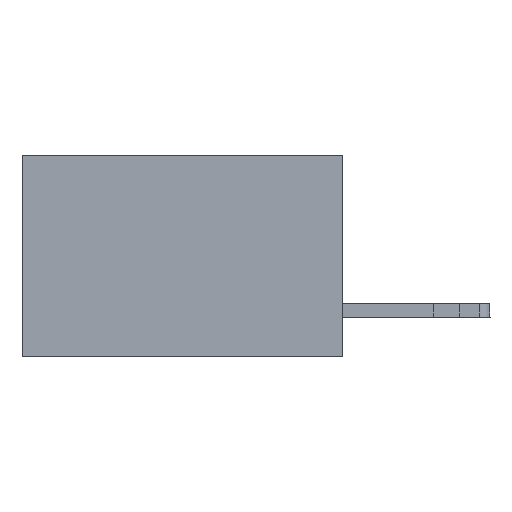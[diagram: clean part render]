
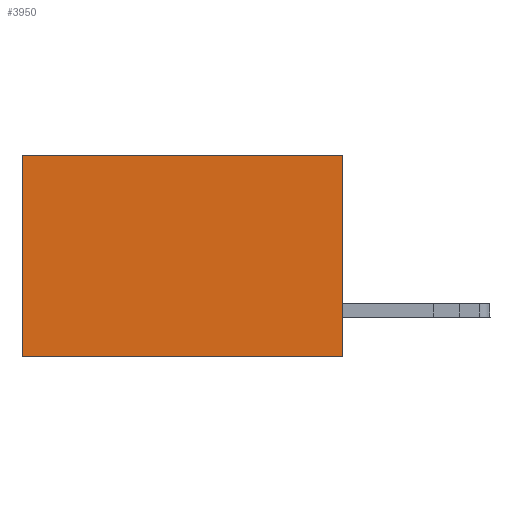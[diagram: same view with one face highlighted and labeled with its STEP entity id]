
A CAD part, left-side view. The second image highlights one B-rep face of the part: STEP entity #3950.
In plain terms, the highlighted planar face has unit normal (-1, 0, 0).
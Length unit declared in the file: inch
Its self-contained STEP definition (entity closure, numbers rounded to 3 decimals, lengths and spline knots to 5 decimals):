
#245 = ORIENTED_EDGE ( 'NONE', *, *, #6672, .F. ) ;
#1164 = DIRECTION ( 'NONE',  ( 0., 0., -1. ) ) ;
#2266 = DIRECTION ( 'NONE',  ( 1., 0., 0. ) ) ;
#2514 = CARTESIAN_POINT ( 'NONE',  ( 0.277, 0., 0. ) ) ;
#2700 = DIRECTION ( 'NONE',  ( 0., 1., 0. ) ) ;
#3463 = VECTOR ( 'NONE', #1164, 39.37008 ) ;
#3659 = EDGE_CURVE ( 'NONE', #6729, #17856, #12805, .T. ) ;
#3688 = EDGE_CURVE ( 'NONE', #8222, #17856, #14069, .T. ) ;
#3950 = ADVANCED_FACE ( 'NONE', ( #10992 ), #16652, .F. ) ;
#4172 = DIRECTION ( 'NONE',  ( 0., 1., 0. ) ) ;
#4713 = EDGE_LOOP ( 'NONE', ( #12100, #17910, #245, #5260 ) ) ;
#5231 = AXIS2_PLACEMENT_3D ( 'NONE', #12423, #2266, #8115 ) ;
#5260 = ORIENTED_EDGE ( 'NONE', *, *, #6637, .T. ) ;
#5488 = CARTESIAN_POINT ( 'NONE',  ( 0.277, 0., 0. ) ) ;
#5833 = VECTOR ( 'NONE', #11285, 39.37008 ) ;
#6637 = EDGE_CURVE ( 'NONE', #10083, #8222, #8464, .T. ) ;
#6672 = EDGE_CURVE ( 'NONE', #10083, #6729, #9715, .T. ) ;
#6729 = VERTEX_POINT ( 'NONE', #18621 ) ;
#6785 = CARTESIAN_POINT ( 'NONE',  ( 0.277, 0.59, -0.37 ) ) ;
#7153 = CARTESIAN_POINT ( 'NONE',  ( 0.277, 0., -0.37 ) ) ;
#8115 = DIRECTION ( 'NONE',  ( 0., 0., -1. ) ) ;
#8222 = VERTEX_POINT ( 'NONE', #11719 ) ;
#8464 = LINE ( 'NONE', #5488, #10498 ) ;
#9715 = LINE ( 'NONE', #18527, #3463 ) ;
#10083 = VERTEX_POINT ( 'NONE', #2514 ) ;
#10498 = VECTOR ( 'NONE', #2700, 39.37008 ) ;
#10992 = FACE_OUTER_BOUND ( 'NONE', #4713, .T. ) ;
#11285 = DIRECTION ( 'NONE',  ( 0., 0., -1. ) ) ;
#11651 = VECTOR ( 'NONE', #4172, 39.37008 ) ;
#11719 = CARTESIAN_POINT ( 'NONE',  ( 0.277, 0.59, 0. ) ) ;
#12100 = ORIENTED_EDGE ( 'NONE', *, *, #3688, .T. ) ;
#12423 = CARTESIAN_POINT ( 'NONE',  ( 0.277, 0., -0.37 ) ) ;
#12805 = LINE ( 'NONE', #7153, #11651 ) ;
#14069 = LINE ( 'NONE', #6785, #5833 ) ;
#15813 = CARTESIAN_POINT ( 'NONE',  ( 0.277, 0.59, -0.37 ) ) ;
#16652 = PLANE ( 'NONE',  #5231 ) ;
#17856 = VERTEX_POINT ( 'NONE', #15813 ) ;
#17910 = ORIENTED_EDGE ( 'NONE', *, *, #3659, .F. ) ;
#18527 = CARTESIAN_POINT ( 'NONE',  ( 0.277, 0., -0.37 ) ) ;
#18621 = CARTESIAN_POINT ( 'NONE',  ( 0.277, 0., -0.37 ) ) ;
